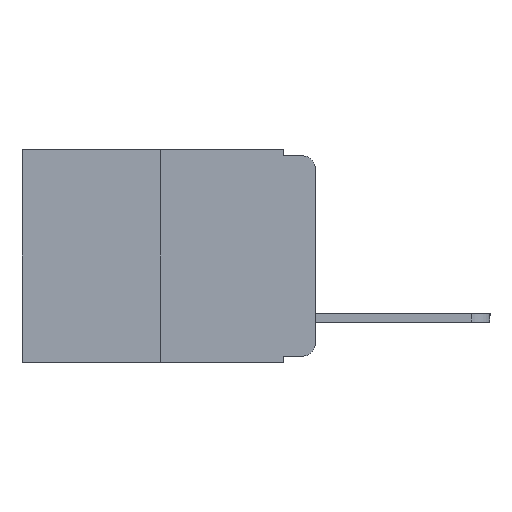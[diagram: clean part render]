
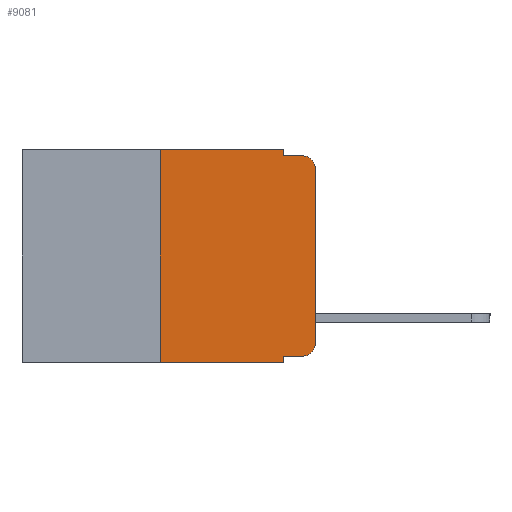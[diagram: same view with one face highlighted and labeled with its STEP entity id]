
A CAD part, left-side view. The second image highlights one B-rep face of the part: STEP entity #9081.
In plain terms, the highlighted planar face has unit normal (-1, 0, 0).
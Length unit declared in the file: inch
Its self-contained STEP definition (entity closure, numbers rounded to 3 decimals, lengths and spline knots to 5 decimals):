
#43 = DIRECTION ( 'NONE',  ( 0., 0., 1. ) ) ;
#243 = LINE ( 'NONE', #7188, #3418 ) ;
#249 = AXIS2_PLACEMENT_3D ( 'NONE', #10988, #4196, #11950 ) ;
#519 = VERTEX_POINT ( 'NONE', #5505 ) ;
#807 = LINE ( 'NONE', #13227, #10420 ) ;
#986 = ORIENTED_EDGE ( 'NONE', *, *, #12431, .F. ) ;
#1019 = VERTEX_POINT ( 'NONE', #11088 ) ;
#1361 = EDGE_CURVE ( 'NONE', #9003, #11209, #13716, .T. ) ;
#1392 = VECTOR ( 'NONE', #9314, 39.37008 ) ;
#1681 = LINE ( 'NONE', #12988, #12782 ) ;
#1774 = ORIENTED_EDGE ( 'NONE', *, *, #10304, .T. ) ;
#1883 = VERTEX_POINT ( 'NONE', #12132 ) ;
#2006 = CARTESIAN_POINT ( 'NONE',  ( 0., 0.051, -0.333 ) ) ;
#2159 = ORIENTED_EDGE ( 'NONE', *, *, #3152, .T. ) ;
#3152 = EDGE_CURVE ( 'NONE', #4038, #9003, #9535, .T. ) ;
#3418 = VECTOR ( 'NONE', #13406, 39.37008 ) ;
#3536 = CIRCLE ( 'NONE', #249, 0.02 ) ;
#3785 = ORIENTED_EDGE ( 'NONE', *, *, #1361, .T. ) ;
#3938 = EDGE_CURVE ( 'NONE', #7800, #4038, #8854, .T. ) ;
#4038 = VERTEX_POINT ( 'NONE', #9421 ) ;
#4196 = DIRECTION ( 'NONE',  ( -1., 0., 0. ) ) ;
#4284 = CARTESIAN_POINT ( 'NONE',  ( 0., 0.051, 0. ) ) ;
#4412 = EDGE_LOOP ( 'NONE', ( #3785, #6925, #12560, #986, #10253, #12851, #1774, #8041, #10906, #2159 ) ) ;
#4438 = AXIS2_PLACEMENT_3D ( 'NONE', #12619, #10672, #10684 ) ;
#4532 = LINE ( 'NONE', #8183, #1392 ) ;
#4755 = CARTESIAN_POINT ( 'NONE',  ( 0., 0.25, 0. ) ) ;
#4791 = CARTESIAN_POINT ( 'NONE',  ( 0., 0.051, -0.333 ) ) ;
#5240 = CARTESIAN_POINT ( 'NONE',  ( 0., 0.051, -0.01 ) ) ;
#5397 = VERTEX_POINT ( 'NONE', #4284 ) ;
#5497 = DIRECTION ( 'NONE',  ( 0., -1., 0. ) ) ;
#5505 = CARTESIAN_POINT ( 'NONE',  ( 0., 0.051, -0.343 ) ) ;
#5636 = EDGE_CURVE ( 'NONE', #8726, #1019, #243, .T. ) ;
#5973 = FACE_OUTER_BOUND ( 'NONE', #4412, .T. ) ;
#6154 = PLANE ( 'NONE',  #7218 ) ;
#6234 = DIRECTION ( 'NONE',  ( 0., 0., 1. ) ) ;
#6925 = ORIENTED_EDGE ( 'NONE', *, *, #10205, .T. ) ;
#7089 = CARTESIAN_POINT ( 'NONE',  ( 0., 0., -0.313 ) ) ;
#7188 = CARTESIAN_POINT ( 'NONE',  ( 0., 0.051, -0.01 ) ) ;
#7218 = AXIS2_PLACEMENT_3D ( 'NONE', #8502, #13545, #7365 ) ;
#7365 = DIRECTION ( 'NONE',  ( 0., 0., -1. ) ) ;
#7680 = DIRECTION ( 'NONE',  ( 0., 0., -1. ) ) ;
#7800 = VERTEX_POINT ( 'NONE', #2006 ) ;
#7901 = EDGE_CURVE ( 'NONE', #7800, #519, #807, .T. ) ;
#8041 = ORIENTED_EDGE ( 'NONE', *, *, #7901, .F. ) ;
#8183 = CARTESIAN_POINT ( 'NONE',  ( 0., 0.473, 0. ) ) ;
#8502 = CARTESIAN_POINT ( 'NONE',  ( 0., 0.473, 0. ) ) ;
#8726 = VERTEX_POINT ( 'NONE', #5240 ) ;
#8854 = LINE ( 'NONE', #4791, #11862 ) ;
#9003 = VERTEX_POINT ( 'NONE', #7089 ) ;
#9031 = VERTEX_POINT ( 'NONE', #11530 ) ;
#9081 = ADVANCED_FACE ( 'NONE', ( #5973 ), #6154, .F. ) ;
#9255 = DIRECTION ( 'NONE',  ( 0., 0., -1. ) ) ;
#9314 = DIRECTION ( 'NONE',  ( 0., -1., 0. ) ) ;
#9421 = CARTESIAN_POINT ( 'NONE',  ( 0., 0.02, -0.333 ) ) ;
#9535 = CIRCLE ( 'NONE', #4438, 0.02 ) ;
#10205 = EDGE_CURVE ( 'NONE', #11209, #1019, #3536, .T. ) ;
#10253 = ORIENTED_EDGE ( 'NONE', *, *, #13023, .F. ) ;
#10304 = EDGE_CURVE ( 'NONE', #9031, #519, #1681, .T. ) ;
#10420 = VECTOR ( 'NONE', #9255, 39.37008 ) ;
#10672 = DIRECTION ( 'NONE',  ( -1., 0., 0. ) ) ;
#10684 = DIRECTION ( 'NONE',  ( 0., 0., -1. ) ) ;
#10857 = VECTOR ( 'NONE', #6234, 39.37008 ) ;
#10906 = ORIENTED_EDGE ( 'NONE', *, *, #3938, .T. ) ;
#10908 = CARTESIAN_POINT ( 'NONE',  ( 0., 0.051, 0. ) ) ;
#10988 = CARTESIAN_POINT ( 'NONE',  ( 0., 0.02, -0.03 ) ) ;
#11088 = CARTESIAN_POINT ( 'NONE',  ( 0., 0.02, -0.01 ) ) ;
#11209 = VERTEX_POINT ( 'NONE', #12138 ) ;
#11216 = VECTOR ( 'NONE', #43, 39.37008 ) ;
#11229 = VECTOR ( 'NONE', #7680, 39.37008 ) ;
#11530 = CARTESIAN_POINT ( 'NONE',  ( 0., 0.25, -0.343 ) ) ;
#11862 = VECTOR ( 'NONE', #13442, 39.37008 ) ;
#11950 = DIRECTION ( 'NONE',  ( 0., 0., -1. ) ) ;
#12132 = CARTESIAN_POINT ( 'NONE',  ( 0., 0.25, 0. ) ) ;
#12138 = CARTESIAN_POINT ( 'NONE',  ( 0., 0., -0.03 ) ) ;
#12431 = EDGE_CURVE ( 'NONE', #5397, #8726, #13787, .T. ) ;
#12560 = ORIENTED_EDGE ( 'NONE', *, *, #5636, .F. ) ;
#12619 = CARTESIAN_POINT ( 'NONE',  ( 0., 0.02, -0.313 ) ) ;
#12782 = VECTOR ( 'NONE', #5497, 39.37008 ) ;
#12851 = ORIENTED_EDGE ( 'NONE', *, *, #12897, .F. ) ;
#12897 = EDGE_CURVE ( 'NONE', #9031, #1883, #13779, .T. ) ;
#12988 = CARTESIAN_POINT ( 'NONE',  ( 0., 0.473, -0.343 ) ) ;
#13023 = EDGE_CURVE ( 'NONE', #1883, #5397, #4532, .T. ) ;
#13227 = CARTESIAN_POINT ( 'NONE',  ( 0., 0.051, 0. ) ) ;
#13278 = CARTESIAN_POINT ( 'NONE',  ( 0., 0., 0. ) ) ;
#13406 = DIRECTION ( 'NONE',  ( 0., -1., 0. ) ) ;
#13442 = DIRECTION ( 'NONE',  ( 0., -1., 0. ) ) ;
#13545 = DIRECTION ( 'NONE',  ( 1., 0., 0. ) ) ;
#13716 = LINE ( 'NONE', #13278, #10857 ) ;
#13779 = LINE ( 'NONE', #4755, #11216 ) ;
#13787 = LINE ( 'NONE', #10908, #11229 ) ;
